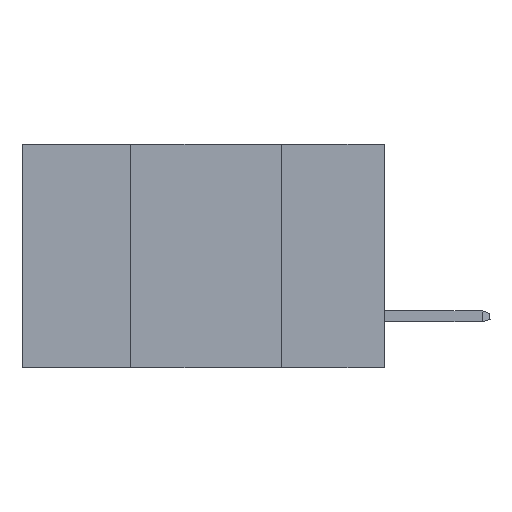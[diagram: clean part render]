
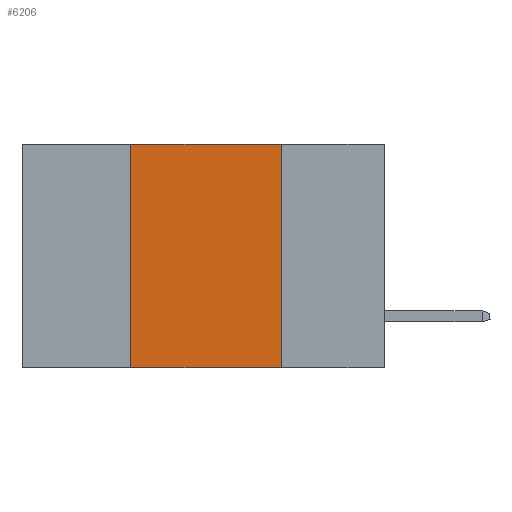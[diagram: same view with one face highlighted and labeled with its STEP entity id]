
A CAD part, left-side view. The second image highlights one B-rep face of the part: STEP entity #6206.
In plain terms, the highlighted planar face has unit normal (-1, 0, 0).
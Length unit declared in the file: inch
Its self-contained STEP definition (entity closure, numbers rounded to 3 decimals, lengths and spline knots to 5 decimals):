
#173 = LINE ( 'NONE', #6840, #4279 ) ;
#198 = ORIENTED_EDGE ( 'NONE', *, *, #2102, .F. ) ;
#225 = VERTEX_POINT ( 'NONE', #6858 ) ;
#421 = CARTESIAN_POINT ( 'NONE',  ( 0., 0.17, 0. ) ) ;
#430 = AXIS2_PLACEMENT_3D ( 'NONE', #4901, #1748, #1881 ) ;
#444 = VERTEX_POINT ( 'NONE', #7873 ) ;
#1404 = EDGE_LOOP ( 'NONE', ( #3251, #198, #3252, #7624 ) ) ;
#1438 = LINE ( 'NONE', #2556, #5782 ) ;
#1748 = DIRECTION ( 'NONE',  ( 1., 0., 0. ) ) ;
#1881 = DIRECTION ( 'NONE',  ( 0., 0., -1. ) ) ;
#2102 = EDGE_CURVE ( 'NONE', #444, #5066, #173, .T. ) ;
#2556 = CARTESIAN_POINT ( 'NONE',  ( 0., 0.6, -0.37 ) ) ;
#3251 = ORIENTED_EDGE ( 'NONE', *, *, #4732, .F. ) ;
#3252 = ORIENTED_EDGE ( 'NONE', *, *, #4838, .F. ) ;
#3946 = VECTOR ( 'NONE', #7186, 39.37008 ) ;
#4279 = VECTOR ( 'NONE', #4777, 39.37008 ) ;
#4489 = VERTEX_POINT ( 'NONE', #6926 ) ;
#4732 = EDGE_CURVE ( 'NONE', #5066, #4489, #8523, .T. ) ;
#4777 = DIRECTION ( 'NONE',  ( 0., -1., 0. ) ) ;
#4838 = EDGE_CURVE ( 'NONE', #225, #444, #6002, .T. ) ;
#4901 = CARTESIAN_POINT ( 'NONE',  ( 0., 0.6, 0. ) ) ;
#5066 = VERTEX_POINT ( 'NONE', #5523 ) ;
#5282 = DIRECTION ( 'NONE',  ( 0., 0., -1. ) ) ;
#5344 = EDGE_CURVE ( 'NONE', #225, #4489, #1438, .T. ) ;
#5523 = CARTESIAN_POINT ( 'NONE',  ( 0., 0.17, 0. ) ) ;
#5562 = DIRECTION ( 'NONE',  ( 0., -1., 0. ) ) ;
#5782 = VECTOR ( 'NONE', #5562, 39.37008 ) ;
#6002 = LINE ( 'NONE', #6473, #3946 ) ;
#6206 = ADVANCED_FACE ( 'NONE', ( #9005 ), #9273, .F. ) ;
#6473 = CARTESIAN_POINT ( 'NONE',  ( 0., 0.42, 0. ) ) ;
#6840 = CARTESIAN_POINT ( 'NONE',  ( 0., 0.6, 0. ) ) ;
#6858 = CARTESIAN_POINT ( 'NONE',  ( 0., 0.42, -0.37 ) ) ;
#6873 = VECTOR ( 'NONE', #5282, 39.37008 ) ;
#6926 = CARTESIAN_POINT ( 'NONE',  ( 0., 0.17, -0.37 ) ) ;
#7186 = DIRECTION ( 'NONE',  ( 0., 0., 1. ) ) ;
#7624 = ORIENTED_EDGE ( 'NONE', *, *, #5344, .T. ) ;
#7873 = CARTESIAN_POINT ( 'NONE',  ( 0., 0.42, 0. ) ) ;
#8523 = LINE ( 'NONE', #421, #6873 ) ;
#9005 = FACE_OUTER_BOUND ( 'NONE', #1404, .T. ) ;
#9273 = PLANE ( 'NONE',  #430 ) ;
